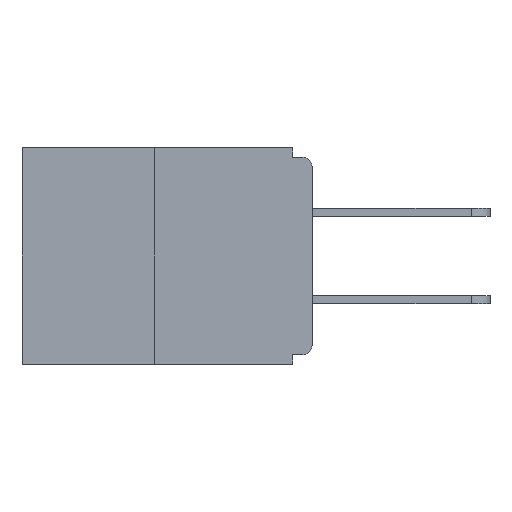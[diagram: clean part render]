
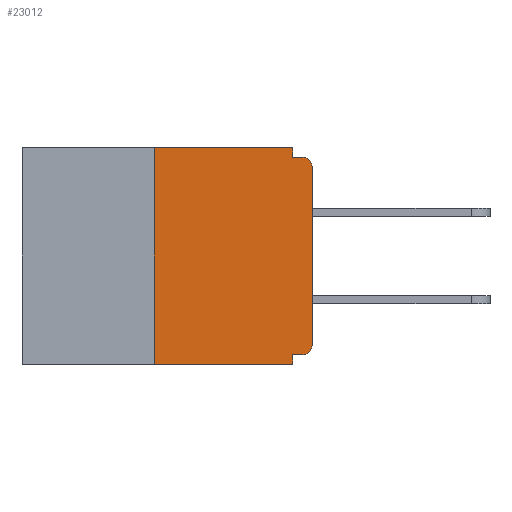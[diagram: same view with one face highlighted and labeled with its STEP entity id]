
A CAD part, left-side view. The second image highlights one B-rep face of the part: STEP entity #23012.
In plain terms, the highlighted planar face has unit normal (-1, 0, 0).
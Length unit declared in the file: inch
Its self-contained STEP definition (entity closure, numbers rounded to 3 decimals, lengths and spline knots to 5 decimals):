
#220 = ORIENTED_EDGE ( 'NONE', *, *, #16447, .F. ) ;
#927 = ORIENTED_EDGE ( 'NONE', *, *, #27561, .T. ) ;
#1325 = VERTEX_POINT ( 'NONE', #9171 ) ;
#1847 = LINE ( 'NONE', #14070, #7627 ) ;
#2016 = LINE ( 'NONE', #18032, #9184 ) ;
#2075 = AXIS2_PLACEMENT_3D ( 'NONE', #25005, #27019, #11849 ) ;
#2722 = DIRECTION ( 'NONE',  ( 0., 1., 0. ) ) ;
#3082 = VERTEX_POINT ( 'NONE', #6983 ) ;
#3629 = LINE ( 'NONE', #14531, #26951 ) ;
#4234 = VECTOR ( 'NONE', #14897, 39.37008 ) ;
#4902 = VERTEX_POINT ( 'NONE', #18695 ) ;
#5371 = VERTEX_POINT ( 'NONE', #9367 ) ;
#5901 = CARTESIAN_POINT ( 'NONE',  ( 0., 0., -0.015 ) ) ;
#5947 = DIRECTION ( 'NONE',  ( -1., 0., 0. ) ) ;
#6086 = FACE_OUTER_BOUND ( 'NONE', #23921, .T. ) ;
#6604 = EDGE_CURVE ( 'NONE', #3082, #19504, #25600, .T. ) ;
#6608 = ORIENTED_EDGE ( 'NONE', *, *, #13450, .F. ) ;
#6902 = LINE ( 'NONE', #5901, #26801 ) ;
#6972 = CARTESIAN_POINT ( 'NONE',  ( 0., 0.031, -0.343 ) ) ;
#6983 = CARTESIAN_POINT ( 'NONE',  ( 0., 0.015, -0.328 ) ) ;
#7627 = VECTOR ( 'NONE', #16291, 39.37008 ) ;
#7766 = CARTESIAN_POINT ( 'NONE',  ( 0., 0.25, 0. ) ) ;
#7918 = CARTESIAN_POINT ( 'NONE',  ( 0., 0.015, -0.03 ) ) ;
#8485 = CARTESIAN_POINT ( 'NONE',  ( 0., 0.46, -0.343 ) ) ;
#9171 = CARTESIAN_POINT ( 'NONE',  ( 0., 0.25, -0.343 ) ) ;
#9184 = VECTOR ( 'NONE', #2722, 39.37008 ) ;
#9275 = VERTEX_POINT ( 'NONE', #7766 ) ;
#9367 = CARTESIAN_POINT ( 'NONE',  ( 0., 0.031, -0.328 ) ) ;
#9583 = VERTEX_POINT ( 'NONE', #27933 ) ;
#10282 = VERTEX_POINT ( 'NONE', #14267 ) ;
#10610 = DIRECTION ( 'NONE',  ( 0., -1., 0. ) ) ;
#10692 = CARTESIAN_POINT ( 'NONE',  ( 0., 0.031, 0. ) ) ;
#11106 = AXIS2_PLACEMENT_3D ( 'NONE', #7918, #16268, #12316 ) ;
#11119 = ORIENTED_EDGE ( 'NONE', *, *, #13577, .F. ) ;
#11849 = DIRECTION ( 'NONE',  ( 0., 0., -1. ) ) ;
#11906 = CIRCLE ( 'NONE', #11106, 0.015 ) ;
#12070 = VERTEX_POINT ( 'NONE', #17339 ) ;
#12268 = VECTOR ( 'NONE', #18389, 39.37008 ) ;
#12316 = DIRECTION ( 'NONE',  ( 0., 0., -1. ) ) ;
#12804 = ORIENTED_EDGE ( 'NONE', *, *, #25681, .F. ) ;
#13039 = EDGE_CURVE ( 'NONE', #9275, #9583, #17644, .T. ) ;
#13450 = EDGE_CURVE ( 'NONE', #9583, #12070, #26868, .T. ) ;
#13577 = EDGE_CURVE ( 'NONE', #1325, #9275, #1847, .T. ) ;
#13833 = CARTESIAN_POINT ( 'NONE',  ( 0., 0., -0.03 ) ) ;
#14059 = CARTESIAN_POINT ( 'NONE',  ( 0., 0.46, 0. ) ) ;
#14070 = CARTESIAN_POINT ( 'NONE',  ( 0., 0.25, 0. ) ) ;
#14267 = CARTESIAN_POINT ( 'NONE',  ( 0., 0.031, -0.343 ) ) ;
#14531 = CARTESIAN_POINT ( 'NONE',  ( 0., 0., 0. ) ) ;
#14897 = DIRECTION ( 'NONE',  ( 0., 0., -1. ) ) ;
#16268 = DIRECTION ( 'NONE',  ( -1., 0., 0. ) ) ;
#16291 = DIRECTION ( 'NONE',  ( 0., 0., 1. ) ) ;
#16447 = EDGE_CURVE ( 'NONE', #3082, #5371, #2016, .T. ) ;
#17339 = CARTESIAN_POINT ( 'NONE',  ( 0., 0.031, -0.015 ) ) ;
#17644 = LINE ( 'NONE', #14059, #24833 ) ;
#18032 = CARTESIAN_POINT ( 'NONE',  ( 0., 0., -0.328 ) ) ;
#18058 = LINE ( 'NONE', #8485, #23881 ) ;
#18389 = DIRECTION ( 'NONE',  ( 0., 0., -1. ) ) ;
#18695 = CARTESIAN_POINT ( 'NONE',  ( 0., 0.015, -0.015 ) ) ;
#18910 = CARTESIAN_POINT ( 'NONE',  ( 0., 0.015, -0.313 ) ) ;
#19197 = DIRECTION ( 'NONE',  ( 0., 0., -1. ) ) ;
#19484 = AXIS2_PLACEMENT_3D ( 'NONE', #18910, #5947, #19197 ) ;
#19504 = VERTEX_POINT ( 'NONE', #23141 ) ;
#20207 = LINE ( 'NONE', #6972, #12268 ) ;
#20415 = DIRECTION ( 'NONE',  ( 0., -1., 0. ) ) ;
#20534 = ORIENTED_EDGE ( 'NONE', *, *, #23832, .T. ) ;
#22362 = ORIENTED_EDGE ( 'NONE', *, *, #6604, .T. ) ;
#22631 = EDGE_CURVE ( 'NONE', #5371, #10282, #20207, .T. ) ;
#23012 = ADVANCED_FACE ( 'NONE', ( #6086 ), #24906, .F. ) ;
#23141 = CARTESIAN_POINT ( 'NONE',  ( 0., 0., -0.313 ) ) ;
#23641 = DIRECTION ( 'NONE',  ( 0., -1., 0. ) ) ;
#23832 = EDGE_CURVE ( 'NONE', #19504, #24880, #3629, .T. ) ;
#23881 = VECTOR ( 'NONE', #10610, 39.37008 ) ;
#23921 = EDGE_LOOP ( 'NONE', ( #24292, #11119, #28001, #27153, #220, #22362, #20534, #927, #12804, #6608 ) ) ;
#23923 = EDGE_CURVE ( 'NONE', #1325, #10282, #18058, .T. ) ;
#24292 = ORIENTED_EDGE ( 'NONE', *, *, #13039, .F. ) ;
#24833 = VECTOR ( 'NONE', #20415, 39.37008 ) ;
#24880 = VERTEX_POINT ( 'NONE', #13833 ) ;
#24906 = PLANE ( 'NONE',  #2075 ) ;
#25005 = CARTESIAN_POINT ( 'NONE',  ( 0., 0.46, 0. ) ) ;
#25572 = DIRECTION ( 'NONE',  ( 0., 0., 1. ) ) ;
#25600 = CIRCLE ( 'NONE', #19484, 0.015 ) ;
#25681 = EDGE_CURVE ( 'NONE', #12070, #4902, #6902, .T. ) ;
#26801 = VECTOR ( 'NONE', #23641, 39.37008 ) ;
#26868 = LINE ( 'NONE', #10692, #4234 ) ;
#26951 = VECTOR ( 'NONE', #25572, 39.37008 ) ;
#27019 = DIRECTION ( 'NONE',  ( 1., 0., 0. ) ) ;
#27153 = ORIENTED_EDGE ( 'NONE', *, *, #22631, .F. ) ;
#27561 = EDGE_CURVE ( 'NONE', #24880, #4902, #11906, .T. ) ;
#27933 = CARTESIAN_POINT ( 'NONE',  ( 0., 0.031, 0. ) ) ;
#28001 = ORIENTED_EDGE ( 'NONE', *, *, #23923, .T. ) ;
